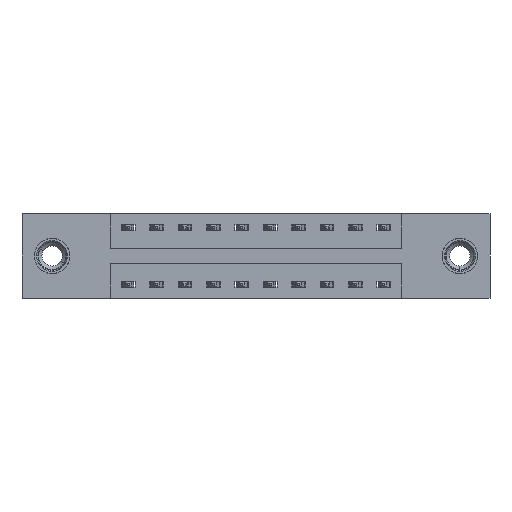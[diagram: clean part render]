
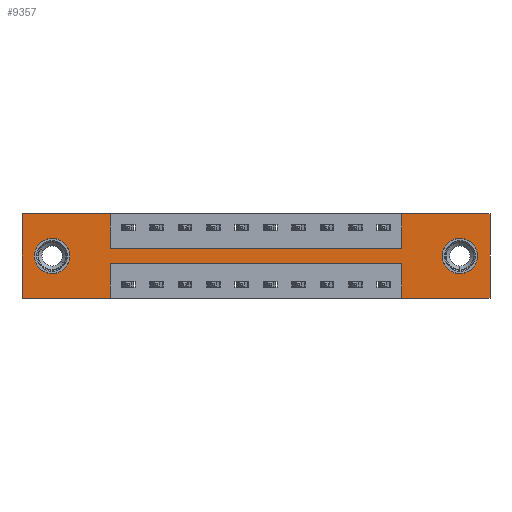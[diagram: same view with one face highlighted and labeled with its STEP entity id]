
A CAD part, front view. The second image highlights one B-rep face of the part: STEP entity #9357.
In plain terms, the highlighted planar face has unit normal (0, -1, 0).
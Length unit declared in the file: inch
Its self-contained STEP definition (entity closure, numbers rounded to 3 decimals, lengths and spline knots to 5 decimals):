
#147 = VERTEX_POINT ( 'NONE', #1394 ) ;
#280 = VERTEX_POINT ( 'NONE', #9837 ) ;
#344 = VECTOR ( 'NONE', #5956, 39.37008 ) ;
#551 = VERTEX_POINT ( 'NONE', #2073 ) ;
#825 = DIRECTION ( 'NONE',  ( 0., 0., 1. ) ) ;
#904 = LINE ( 'NONE', #3505, #3127 ) ;
#1064 = AXIS2_PLACEMENT_3D ( 'NONE', #3371, #1454, #3260 ) ;
#1093 = LINE ( 'NONE', #11313, #6674 ) ;
#1165 = CIRCLE ( 'NONE', #7424, 0.078 ) ;
#1273 = LINE ( 'NONE', #8075, #10697 ) ;
#1322 = AXIS2_PLACEMENT_3D ( 'NONE', #5064, #3183, #5190 ) ;
#1390 = CARTESIAN_POINT ( 'NONE',  ( 2.06, 0., -0.37 ) ) ;
#1394 = CARTESIAN_POINT ( 'NONE',  ( 0.1325, 0., -0.107 ) ) ;
#1454 = DIRECTION ( 'NONE',  ( 0., 1., 0. ) ) ;
#1651 = CARTESIAN_POINT ( 'NONE',  ( 0.3875, 0., 0. ) ) ;
#1738 = VERTEX_POINT ( 'NONE', #7383 ) ;
#2073 = CARTESIAN_POINT ( 'NONE',  ( 1.6725, 0., -0.15 ) ) ;
#2087 = ORIENTED_EDGE ( 'NONE', *, *, #8584, .F. ) ;
#2272 = VECTOR ( 'NONE', #5173, 39.37008 ) ;
#2377 = EDGE_CURVE ( 'NONE', #11164, #280, #1093, .T. ) ;
#2488 = VECTOR ( 'NONE', #8147, 39.37008 ) ;
#2519 = FACE_BOUND ( 'NONE', #10325, .T. ) ;
#2624 = VERTEX_POINT ( 'NONE', #1651 ) ;
#2645 = LINE ( 'NONE', #5570, #3732 ) ;
#2670 = VECTOR ( 'NONE', #10355, 39.37008 ) ;
#2704 = ORIENTED_EDGE ( 'NONE', *, *, #7826, .T. ) ;
#2763 = VECTOR ( 'NONE', #5979, 39.37008 ) ;
#2980 = ORIENTED_EDGE ( 'NONE', *, *, #11284, .F. ) ;
#2990 = CARTESIAN_POINT ( 'NONE',  ( 1.6725, 0., -0.22 ) ) ;
#3005 = CARTESIAN_POINT ( 'NONE',  ( 0.3875, 0., -0.22 ) ) ;
#3089 = EDGE_CURVE ( 'NONE', #7470, #6622, #9480, .T. ) ;
#3127 = VECTOR ( 'NONE', #12009, 39.37008 ) ;
#3183 = DIRECTION ( 'NONE',  ( 0., 1., 0. ) ) ;
#3260 = DIRECTION ( 'NONE',  ( 0., 0., 1. ) ) ;
#3293 = LINE ( 'NONE', #7910, #2272 ) ;
#3303 = CARTESIAN_POINT ( 'NONE',  ( 2.06, 0., 0. ) ) ;
#3371 = CARTESIAN_POINT ( 'NONE',  ( 0.1325, 0., -0.185 ) ) ;
#3444 = VECTOR ( 'NONE', #6232, 39.37008 ) ;
#3477 = DIRECTION ( 'NONE',  ( 0., -1., 0. ) ) ;
#3482 = CARTESIAN_POINT ( 'NONE',  ( 0., 0., -0.37 ) ) ;
#3501 = LINE ( 'NONE', #9110, #2488 ) ;
#3505 = CARTESIAN_POINT ( 'NONE',  ( 0.3875, 0., -0.15 ) ) ;
#3524 = ORIENTED_EDGE ( 'NONE', *, *, #8862, .F. ) ;
#3732 = VECTOR ( 'NONE', #825, 39.37008 ) ;
#3770 = CARTESIAN_POINT ( 'NONE',  ( 0.1325, 0., -0.263 ) ) ;
#3835 = CARTESIAN_POINT ( 'NONE',  ( 1.6725, 0., 0. ) ) ;
#4022 = VECTOR ( 'NONE', #7193, 39.37008 ) ;
#4075 = CARTESIAN_POINT ( 'NONE',  ( 0., 0., 0. ) ) ;
#4238 = DIRECTION ( 'NONE',  ( 0., 0., 1. ) ) ;
#4313 = EDGE_CURVE ( 'NONE', #2624, #7284, #6178, .T. ) ;
#4395 = EDGE_CURVE ( 'NONE', #147, #11712, #4603, .T. ) ;
#4603 = CIRCLE ( 'NONE', #1064, 0.078 ) ;
#4688 = LINE ( 'NONE', #11107, #8224 ) ;
#4855 = CARTESIAN_POINT ( 'NONE',  ( 1.9275, 0., -0.107 ) ) ;
#4876 = CARTESIAN_POINT ( 'NONE',  ( 1.9275, 0., -0.185 ) ) ;
#5064 = CARTESIAN_POINT ( 'NONE',  ( 1.9275, 0., -0.185 ) ) ;
#5173 = DIRECTION ( 'NONE',  ( 0., 0., 1. ) ) ;
#5190 = DIRECTION ( 'NONE',  ( 0., 0., -1. ) ) ;
#5263 = CARTESIAN_POINT ( 'NONE',  ( 0.3875, 0., 0. ) ) ;
#5287 = AXIS2_PLACEMENT_3D ( 'NONE', #6409, #3477, #9139 ) ;
#5460 = VERTEX_POINT ( 'NONE', #11951 ) ;
#5471 = CARTESIAN_POINT ( 'NONE',  ( 0.1325, 0., -0.185 ) ) ;
#5502 = FACE_OUTER_BOUND ( 'NONE', #10838, .T. ) ;
#5570 = CARTESIAN_POINT ( 'NONE',  ( 1.6725, 0., -0.37 ) ) ;
#5589 = ORIENTED_EDGE ( 'NONE', *, *, #4313, .F. ) ;
#5760 = DIRECTION ( 'NONE',  ( 0., 0., 1. ) ) ;
#5864 = CARTESIAN_POINT ( 'NONE',  ( 0.3875, 0., -0.15 ) ) ;
#5956 = DIRECTION ( 'NONE',  ( 1., 0., 0. ) ) ;
#5979 = DIRECTION ( 'NONE',  ( 1., 0., 0. ) ) ;
#6020 = EDGE_CURVE ( 'NONE', #8297, #11075, #9436, .T. ) ;
#6138 = VERTEX_POINT ( 'NONE', #3303 ) ;
#6178 = LINE ( 'NONE', #5263, #3444 ) ;
#6232 = DIRECTION ( 'NONE',  ( 0., 0., -1. ) ) ;
#6318 = ORIENTED_EDGE ( 'NONE', *, *, #6020, .F. ) ;
#6409 = CARTESIAN_POINT ( 'NONE',  ( 0., 0., -0.37 ) ) ;
#6558 = EDGE_CURVE ( 'NONE', #551, #9516, #3293, .T. ) ;
#6587 = DIRECTION ( 'NONE',  ( 0., 0., -1. ) ) ;
#6622 = VERTEX_POINT ( 'NONE', #10211 ) ;
#6674 = VECTOR ( 'NONE', #5760, 39.37008 ) ;
#7096 = EDGE_CURVE ( 'NONE', #6138, #7470, #3501, .T. ) ;
#7193 = DIRECTION ( 'NONE',  ( -1., 0., 0. ) ) ;
#7284 = VERTEX_POINT ( 'NONE', #5864 ) ;
#7383 = CARTESIAN_POINT ( 'NONE',  ( 0.3875, 0., -0.37 ) ) ;
#7424 = AXIS2_PLACEMENT_3D ( 'NONE', #5471, #8934, #4238 ) ;
#7470 = VERTEX_POINT ( 'NONE', #1390 ) ;
#7826 = EDGE_CURVE ( 'NONE', #11961, #5460, #8550, .T. ) ;
#7910 = CARTESIAN_POINT ( 'NONE',  ( 1.6725, 0., 0. ) ) ;
#8075 = CARTESIAN_POINT ( 'NONE',  ( 0., 0., -0.37 ) ) ;
#8128 = CARTESIAN_POINT ( 'NONE',  ( 0., 0., -0.37 ) ) ;
#8147 = DIRECTION ( 'NONE',  ( 0., 0., -1. ) ) ;
#8224 = VECTOR ( 'NONE', #6587, 39.37008 ) ;
#8297 = VERTEX_POINT ( 'NONE', #2990 ) ;
#8550 = CIRCLE ( 'NONE', #1322, 0.078 ) ;
#8584 = EDGE_CURVE ( 'NONE', #7284, #551, #904, .T. ) ;
#8782 = AXIS2_PLACEMENT_3D ( 'NONE', #4876, #11129, #10145 ) ;
#8862 = EDGE_CURVE ( 'NONE', #1738, #11164, #1273, .T. ) ;
#8905 = ORIENTED_EDGE ( 'NONE', *, *, #2377, .F. ) ;
#8934 = DIRECTION ( 'NONE',  ( 0., 1., 0. ) ) ;
#8962 = PLANE ( 'NONE',  #5287 ) ;
#9110 = CARTESIAN_POINT ( 'NONE',  ( 2.06, 0., 0. ) ) ;
#9114 = ORIENTED_EDGE ( 'NONE', *, *, #3089, .F. ) ;
#9139 = DIRECTION ( 'NONE',  ( 0., 0., -1. ) ) ;
#9320 = ORIENTED_EDGE ( 'NONE', *, *, #11299, .F. ) ;
#9357 = ADVANCED_FACE ( 'NONE', ( #2519, #11757, #5502 ), #8962, .T. ) ;
#9436 = LINE ( 'NONE', #3005, #2670 ) ;
#9480 = LINE ( 'NONE', #3482, #4022 ) ;
#9516 = VERTEX_POINT ( 'NONE', #3835 ) ;
#9556 = CIRCLE ( 'NONE', #8782, 0.078 ) ;
#9611 = LINE ( 'NONE', #10515, #344 ) ;
#9646 = DIRECTION ( 'NONE',  ( -1., 0., 0. ) ) ;
#9837 = CARTESIAN_POINT ( 'NONE',  ( 0., 0., 0. ) ) ;
#10076 = ORIENTED_EDGE ( 'NONE', *, *, #4395, .T. ) ;
#10145 = DIRECTION ( 'NONE',  ( 0., 0., -1. ) ) ;
#10169 = ORIENTED_EDGE ( 'NONE', *, *, #10227, .T. ) ;
#10211 = CARTESIAN_POINT ( 'NONE',  ( 1.6725, 0., -0.37 ) ) ;
#10227 = EDGE_CURVE ( 'NONE', #11712, #147, #1165, .T. ) ;
#10246 = EDGE_LOOP ( 'NONE', ( #10076, #10169 ) ) ;
#10325 = EDGE_LOOP ( 'NONE', ( #2704, #10872 ) ) ;
#10328 = EDGE_CURVE ( 'NONE', #5460, #11961, #9556, .T. ) ;
#10331 = ORIENTED_EDGE ( 'NONE', *, *, #6558, .F. ) ;
#10355 = DIRECTION ( 'NONE',  ( -1., 0., 0. ) ) ;
#10514 = EDGE_CURVE ( 'NONE', #9516, #6138, #10718, .T. ) ;
#10515 = CARTESIAN_POINT ( 'NONE',  ( 0., 0., 0. ) ) ;
#10693 = EDGE_CURVE ( 'NONE', #280, #2624, #9611, .T. ) ;
#10697 = VECTOR ( 'NONE', #9646, 39.37008 ) ;
#10699 = ORIENTED_EDGE ( 'NONE', *, *, #10693, .F. ) ;
#10718 = LINE ( 'NONE', #4075, #2763 ) ;
#10818 = ORIENTED_EDGE ( 'NONE', *, *, #10514, .F. ) ;
#10832 = ORIENTED_EDGE ( 'NONE', *, *, #7096, .F. ) ;
#10838 = EDGE_LOOP ( 'NONE', ( #2980, #6318, #9320, #9114, #10832, #10818, #10331, #2087, #5589, #10699, #8905, #3524 ) ) ;
#10872 = ORIENTED_EDGE ( 'NONE', *, *, #10328, .T. ) ;
#11075 = VERTEX_POINT ( 'NONE', #11709 ) ;
#11107 = CARTESIAN_POINT ( 'NONE',  ( 0.3875, 0., -0.37 ) ) ;
#11129 = DIRECTION ( 'NONE',  ( 0., 1., 0. ) ) ;
#11164 = VERTEX_POINT ( 'NONE', #8128 ) ;
#11284 = EDGE_CURVE ( 'NONE', #11075, #1738, #4688, .T. ) ;
#11299 = EDGE_CURVE ( 'NONE', #6622, #8297, #2645, .T. ) ;
#11313 = CARTESIAN_POINT ( 'NONE',  ( 0., 0., 0. ) ) ;
#11709 = CARTESIAN_POINT ( 'NONE',  ( 0.3875, 0., -0.22 ) ) ;
#11712 = VERTEX_POINT ( 'NONE', #3770 ) ;
#11757 = FACE_BOUND ( 'NONE', #10246, .T. ) ;
#11951 = CARTESIAN_POINT ( 'NONE',  ( 1.9275, 0., -0.263 ) ) ;
#11961 = VERTEX_POINT ( 'NONE', #4855 ) ;
#12009 = DIRECTION ( 'NONE',  ( 1., 0., 0. ) ) ;
